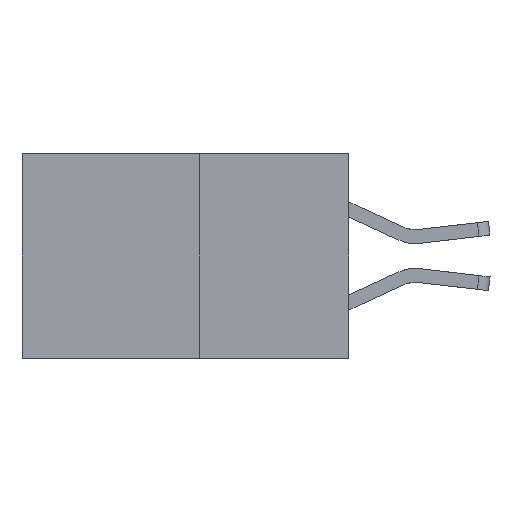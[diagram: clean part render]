
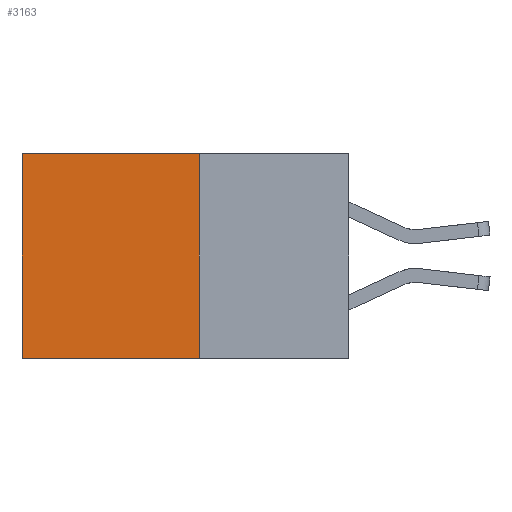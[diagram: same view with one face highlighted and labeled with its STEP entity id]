
A CAD part, left-side view. The second image highlights one B-rep face of the part: STEP entity #3163.
In plain terms, the highlighted planar face has unit normal (-1, 0, 0).
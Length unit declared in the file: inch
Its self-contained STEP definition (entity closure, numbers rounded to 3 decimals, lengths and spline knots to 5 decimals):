
#64 = VERTEX_POINT ( 'NONE', #832 ) ;
#560 = DIRECTION ( 'NONE',  ( 0., 0., -1. ) ) ;
#580 = EDGE_CURVE ( 'NONE', #2283, #5420, #9163, .T. ) ;
#832 = CARTESIAN_POINT ( 'NONE',  ( 0.277, 0.27, 0. ) ) ;
#1339 = ORIENTED_EDGE ( 'NONE', *, *, #580, .T. ) ;
#1771 = DIRECTION ( 'NONE',  ( 0., 0., -1. ) ) ;
#1962 = VECTOR ( 'NONE', #11084, 39.37008 ) ;
#1985 = LINE ( 'NONE', #7783, #10660 ) ;
#2234 = VERTEX_POINT ( 'NONE', #9111 ) ;
#2283 = VERTEX_POINT ( 'NONE', #8427 ) ;
#3163 = ADVANCED_FACE ( 'NONE', ( #7824 ), #10214, .F. ) ;
#3495 = DIRECTION ( 'NONE',  ( 0., 0., -1. ) ) ;
#3682 = ORIENTED_EDGE ( 'NONE', *, *, #10006, .F. ) ;
#3740 = CARTESIAN_POINT ( 'NONE',  ( 0.277, 0.27, -0.37 ) ) ;
#4056 = DIRECTION ( 'NONE',  ( 0., 1., 0. ) ) ;
#4220 = EDGE_LOOP ( 'NONE', ( #1339, #3682, #8960, #10962 ) ) ;
#4386 = LINE ( 'NONE', #3740, #1962 ) ;
#4669 = CARTESIAN_POINT ( 'NONE',  ( 0.277, 0.59, -0.37 ) ) ;
#5420 = VERTEX_POINT ( 'NONE', #4669 ) ;
#5937 = AXIS2_PLACEMENT_3D ( 'NONE', #10970, #6217, #560 ) ;
#6217 = DIRECTION ( 'NONE',  ( 1., 0., 0. ) ) ;
#7783 = CARTESIAN_POINT ( 'NONE',  ( 0.277, 0.27, -0.37 ) ) ;
#7824 = FACE_OUTER_BOUND ( 'NONE', #4220, .T. ) ;
#8098 = EDGE_CURVE ( 'NONE', #64, #2234, #1985, .T. ) ;
#8322 = CARTESIAN_POINT ( 'NONE',  ( 0.277, 0.27, 0. ) ) ;
#8427 = CARTESIAN_POINT ( 'NONE',  ( 0.277, 0.59, 0. ) ) ;
#8575 = CARTESIAN_POINT ( 'NONE',  ( 0.277, 0.59, -0.37 ) ) ;
#8751 = VECTOR ( 'NONE', #4056, 39.37008 ) ;
#8929 = VECTOR ( 'NONE', #1771, 39.37008 ) ;
#8960 = ORIENTED_EDGE ( 'NONE', *, *, #8098, .F. ) ;
#9111 = CARTESIAN_POINT ( 'NONE',  ( 0.277, 0.27, -0.37 ) ) ;
#9163 = LINE ( 'NONE', #8575, #8929 ) ;
#10006 = EDGE_CURVE ( 'NONE', #2234, #5420, #4386, .T. ) ;
#10214 = PLANE ( 'NONE',  #5937 ) ;
#10483 = EDGE_CURVE ( 'NONE', #64, #2283, #10988, .T. ) ;
#10660 = VECTOR ( 'NONE', #3495, 39.37008 ) ;
#10962 = ORIENTED_EDGE ( 'NONE', *, *, #10483, .T. ) ;
#10970 = CARTESIAN_POINT ( 'NONE',  ( 0.277, 0.27, -0.37 ) ) ;
#10988 = LINE ( 'NONE', #8322, #8751 ) ;
#11084 = DIRECTION ( 'NONE',  ( 0., 1., 0. ) ) ;
